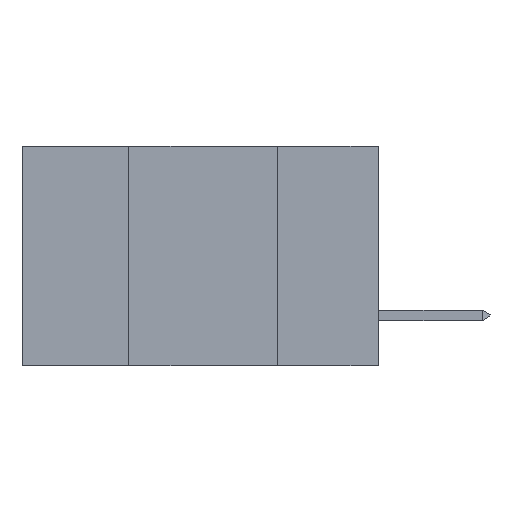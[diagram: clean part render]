
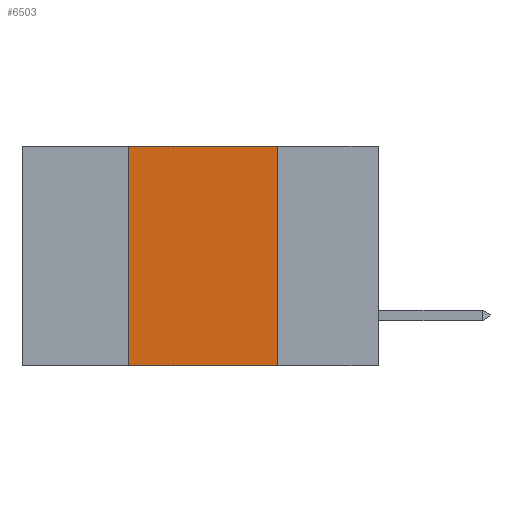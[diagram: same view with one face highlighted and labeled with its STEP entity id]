
A CAD part, left-side view. The second image highlights one B-rep face of the part: STEP entity #6503.
In plain terms, the highlighted planar face has unit normal (-1, 0, 0).
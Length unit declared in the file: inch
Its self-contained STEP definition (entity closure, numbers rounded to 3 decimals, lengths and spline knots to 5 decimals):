
#350 = DIRECTION ( 'NONE',  ( 0., -1., 0. ) ) ;
#446 = DIRECTION ( 'NONE',  ( 0., 0., -1. ) ) ;
#610 = DIRECTION ( 'NONE',  ( 1., 0., 0. ) ) ;
#1525 = CARTESIAN_POINT ( 'NONE',  ( 0., 0.42, -0.37 ) ) ;
#2056 = ORIENTED_EDGE ( 'NONE', *, *, #21832, .F. ) ;
#2936 = LINE ( 'NONE', #15516, #7321 ) ;
#3037 = CARTESIAN_POINT ( 'NONE',  ( 0., 0.17, 0. ) ) ;
#3093 = ORIENTED_EDGE ( 'NONE', *, *, #3099, .T. ) ;
#3099 = EDGE_CURVE ( 'NONE', #22538, #21482, #2936, .T. ) ;
#3472 = LINE ( 'NONE', #3037, #5280 ) ;
#3823 = LINE ( 'NONE', #14894, #25231 ) ;
#4675 = CARTESIAN_POINT ( 'NONE',  ( 0., 0.17, -0.37 ) ) ;
#4819 = EDGE_CURVE ( 'NONE', #14338, #21425, #3823, .T. ) ;
#5280 = VECTOR ( 'NONE', #14662, 39.37008 ) ;
#6503 = ADVANCED_FACE ( 'NONE', ( #17183 ), #21857, .F. ) ;
#6885 = CARTESIAN_POINT ( 'NONE',  ( 0., 0.17, 0. ) ) ;
#7321 = VECTOR ( 'NONE', #11670, 39.37008 ) ;
#7379 = ORIENTED_EDGE ( 'NONE', *, *, #4819, .F. ) ;
#8270 = CARTESIAN_POINT ( 'NONE',  ( 0., 0.42, 0. ) ) ;
#11670 = DIRECTION ( 'NONE',  ( 0., -1., 0. ) ) ;
#11683 = EDGE_LOOP ( 'NONE', ( #2056, #7379, #23858, #3093 ) ) ;
#13301 = AXIS2_PLACEMENT_3D ( 'NONE', #18276, #610, #446 ) ;
#14338 = VERTEX_POINT ( 'NONE', #20508 ) ;
#14662 = DIRECTION ( 'NONE',  ( 0., 0., -1. ) ) ;
#14894 = CARTESIAN_POINT ( 'NONE',  ( 0., 0.6, 0. ) ) ;
#15516 = CARTESIAN_POINT ( 'NONE',  ( 0., 0.6, -0.37 ) ) ;
#16177 = LINE ( 'NONE', #8270, #25328 ) ;
#17183 = FACE_OUTER_BOUND ( 'NONE', #11683, .T. ) ;
#18276 = CARTESIAN_POINT ( 'NONE',  ( 0., 0.6, 0. ) ) ;
#20508 = CARTESIAN_POINT ( 'NONE',  ( 0., 0.42, 0. ) ) ;
#21425 = VERTEX_POINT ( 'NONE', #6885 ) ;
#21482 = VERTEX_POINT ( 'NONE', #4675 ) ;
#21832 = EDGE_CURVE ( 'NONE', #21425, #21482, #3472, .T. ) ;
#21857 = PLANE ( 'NONE',  #13301 ) ;
#21932 = DIRECTION ( 'NONE',  ( 0., 0., 1. ) ) ;
#22538 = VERTEX_POINT ( 'NONE', #1525 ) ;
#23858 = ORIENTED_EDGE ( 'NONE', *, *, #24292, .F. ) ;
#24292 = EDGE_CURVE ( 'NONE', #22538, #14338, #16177, .T. ) ;
#25231 = VECTOR ( 'NONE', #350, 39.37008 ) ;
#25328 = VECTOR ( 'NONE', #21932, 39.37008 ) ;
